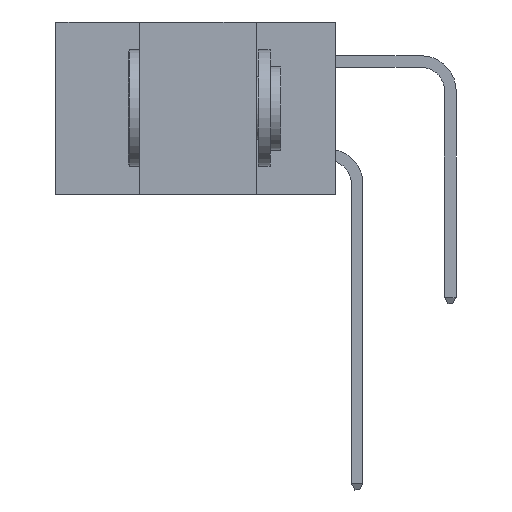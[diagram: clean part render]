
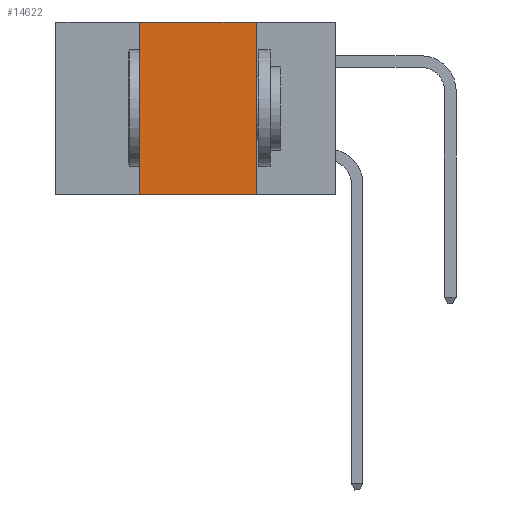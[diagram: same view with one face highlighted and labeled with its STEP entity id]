
A CAD part, left-side view. The second image highlights one B-rep face of the part: STEP entity #14622.
In plain terms, the highlighted planar face has unit normal (-1, 0, 0).
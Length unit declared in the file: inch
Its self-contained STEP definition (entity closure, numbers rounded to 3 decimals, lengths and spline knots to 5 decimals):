
#151 = LINE ( 'NONE', #30848, #4070 ) ;
#1013 = CARTESIAN_POINT ( 'NONE',  ( 0., 0.6, 0. ) ) ;
#1256 = CARTESIAN_POINT ( 'NONE',  ( 0., 0.17, 0. ) ) ;
#1566 = ORIENTED_EDGE ( 'NONE', *, *, #21087, .F. ) ;
#1593 = DIRECTION ( 'NONE',  ( 1., 0., 0. ) ) ;
#2560 = ORIENTED_EDGE ( 'NONE', *, *, #11067, .T. ) ;
#3298 = EDGE_LOOP ( 'NONE', ( #1566, #21430, #23953, #2560 ) ) ;
#4070 = VECTOR ( 'NONE', #12262, 39.37008 ) ;
#4766 = VERTEX_POINT ( 'NONE', #12785 ) ;
#4795 = DIRECTION ( 'NONE',  ( 0., 0., -1. ) ) ;
#5979 = FACE_OUTER_BOUND ( 'NONE', #3298, .T. ) ;
#6873 = VERTEX_POINT ( 'NONE', #10064 ) ;
#8919 = DIRECTION ( 'NONE',  ( 0., -1., 0. ) ) ;
#8942 = VECTOR ( 'NONE', #20739, 39.37008 ) ;
#9370 = VERTEX_POINT ( 'NONE', #1256 ) ;
#10064 = CARTESIAN_POINT ( 'NONE',  ( 0., 0.42, -0.37 ) ) ;
#10790 = CARTESIAN_POINT ( 'NONE',  ( 0., 0.42, 0. ) ) ;
#11067 = EDGE_CURVE ( 'NONE', #6873, #29662, #16300, .T. ) ;
#11429 = DIRECTION ( 'NONE',  ( 0., -1., 0. ) ) ;
#12262 = DIRECTION ( 'NONE',  ( 0., 0., -1. ) ) ;
#12401 = VECTOR ( 'NONE', #8919, 39.37008 ) ;
#12785 = CARTESIAN_POINT ( 'NONE',  ( 0., 0.42, 0. ) ) ;
#13265 = CARTESIAN_POINT ( 'NONE',  ( 0., 0.17, -0.37 ) ) ;
#13703 = VECTOR ( 'NONE', #11429, 39.37008 ) ;
#14622 = ADVANCED_FACE ( 'NONE', ( #5979 ), #15075, .F. ) ;
#15075 = PLANE ( 'NONE',  #31940 ) ;
#16047 = LINE ( 'NONE', #1013, #13703 ) ;
#16300 = LINE ( 'NONE', #26778, #12401 ) ;
#19893 = LINE ( 'NONE', #10790, #8942 ) ;
#20739 = DIRECTION ( 'NONE',  ( 0., 0., 1. ) ) ;
#21087 = EDGE_CURVE ( 'NONE', #9370, #29662, #151, .T. ) ;
#21430 = ORIENTED_EDGE ( 'NONE', *, *, #25388, .F. ) ;
#23953 = ORIENTED_EDGE ( 'NONE', *, *, #27167, .F. ) ;
#25388 = EDGE_CURVE ( 'NONE', #4766, #9370, #16047, .T. ) ;
#26778 = CARTESIAN_POINT ( 'NONE',  ( 0., 0.6, -0.37 ) ) ;
#27167 = EDGE_CURVE ( 'NONE', #6873, #4766, #19893, .T. ) ;
#27602 = CARTESIAN_POINT ( 'NONE',  ( 0., 0.6, 0. ) ) ;
#29662 = VERTEX_POINT ( 'NONE', #13265 ) ;
#30848 = CARTESIAN_POINT ( 'NONE',  ( 0., 0.17, 0. ) ) ;
#31940 = AXIS2_PLACEMENT_3D ( 'NONE', #27602, #1593, #4795 ) ;
